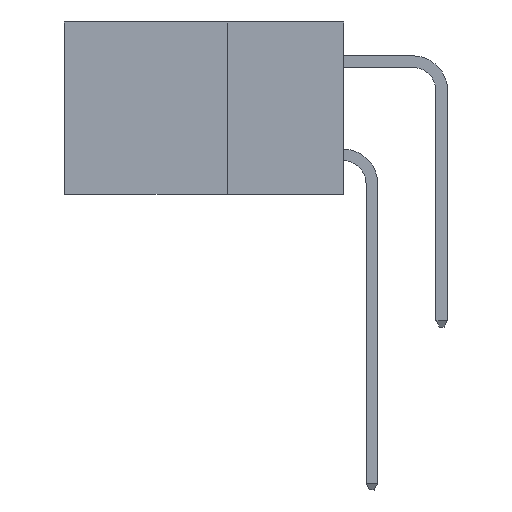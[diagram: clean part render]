
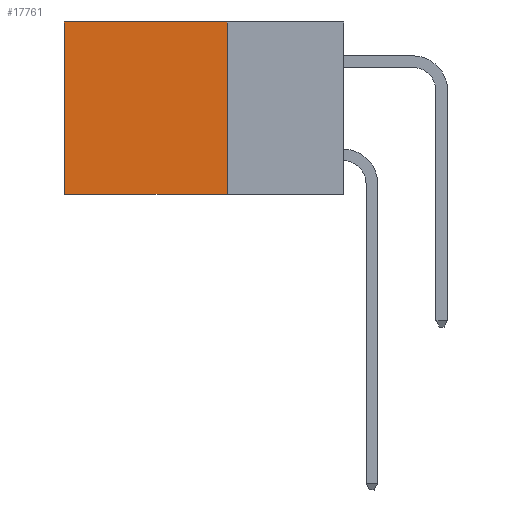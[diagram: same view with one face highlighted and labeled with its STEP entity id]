
A CAD part, left-side view. The second image highlights one B-rep face of the part: STEP entity #17761.
In plain terms, the highlighted planar face has unit normal (-1, 0, 0).
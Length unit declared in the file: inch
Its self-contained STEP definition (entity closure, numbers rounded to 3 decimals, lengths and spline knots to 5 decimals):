
#552 = CARTESIAN_POINT ( 'NONE',  ( 0.298, 0.25, 0. ) ) ;
#1057 = VERTEX_POINT ( 'NONE', #21336 ) ;
#1118 = DIRECTION ( 'NONE',  ( 1., 0., 0. ) ) ;
#1764 = EDGE_CURVE ( 'NONE', #9194, #1057, #7791, .T. ) ;
#2423 = ORIENTED_EDGE ( 'NONE', *, *, #3256, .T. ) ;
#2697 = VECTOR ( 'NONE', #17748, 39.37008 ) ;
#3256 = EDGE_CURVE ( 'NONE', #9194, #3836, #3509, .T. ) ;
#3295 = VERTEX_POINT ( 'NONE', #19093 ) ;
#3509 = LINE ( 'NONE', #22811, #17253 ) ;
#3836 = VERTEX_POINT ( 'NONE', #22171 ) ;
#5057 = ORIENTED_EDGE ( 'NONE', *, *, #16269, .T. ) ;
#5183 = VECTOR ( 'NONE', #11654, 39.37008 ) ;
#5427 = DIRECTION ( 'NONE',  ( 0., 0., -1. ) ) ;
#6033 = CARTESIAN_POINT ( 'NONE',  ( 0.298, 0.25, -0.37 ) ) ;
#6634 = PLANE ( 'NONE',  #7722 ) ;
#7531 = LINE ( 'NONE', #20784, #8765 ) ;
#7722 = AXIS2_PLACEMENT_3D ( 'NONE', #10492, #1118, #22138 ) ;
#7791 = LINE ( 'NONE', #552, #2697 ) ;
#8765 = VECTOR ( 'NONE', #5427, 39.37008 ) ;
#9194 = VERTEX_POINT ( 'NONE', #12141 ) ;
#10492 = CARTESIAN_POINT ( 'NONE',  ( 0.298, 0.25, 0. ) ) ;
#11654 = DIRECTION ( 'NONE',  ( 0., 1., 0. ) ) ;
#12141 = CARTESIAN_POINT ( 'NONE',  ( 0.298, 0.25, 0. ) ) ;
#15943 = EDGE_LOOP ( 'NONE', ( #5057, #19621, #18711, #2423 ) ) ;
#16269 = EDGE_CURVE ( 'NONE', #3836, #3295, #7531, .T. ) ;
#17253 = VECTOR ( 'NONE', #19170, 39.37008 ) ;
#17748 = DIRECTION ( 'NONE',  ( 0., 0., -1. ) ) ;
#17761 = ADVANCED_FACE ( 'NONE', ( #23853 ), #6634, .F. ) ;
#18711 = ORIENTED_EDGE ( 'NONE', *, *, #1764, .F. ) ;
#19093 = CARTESIAN_POINT ( 'NONE',  ( 0.298, 0.6, -0.37 ) ) ;
#19170 = DIRECTION ( 'NONE',  ( 0., 1., 0. ) ) ;
#19252 = LINE ( 'NONE', #6033, #5183 ) ;
#19621 = ORIENTED_EDGE ( 'NONE', *, *, #21217, .F. ) ;
#20784 = CARTESIAN_POINT ( 'NONE',  ( 0.298, 0.6, 0. ) ) ;
#21217 = EDGE_CURVE ( 'NONE', #1057, #3295, #19252, .T. ) ;
#21336 = CARTESIAN_POINT ( 'NONE',  ( 0.298, 0.25, -0.37 ) ) ;
#22138 = DIRECTION ( 'NONE',  ( 0., 0., -1. ) ) ;
#22171 = CARTESIAN_POINT ( 'NONE',  ( 0.298, 0.6, 0. ) ) ;
#22811 = CARTESIAN_POINT ( 'NONE',  ( 0.298, 0.25, 0. ) ) ;
#23853 = FACE_OUTER_BOUND ( 'NONE', #15943, .T. ) ;
